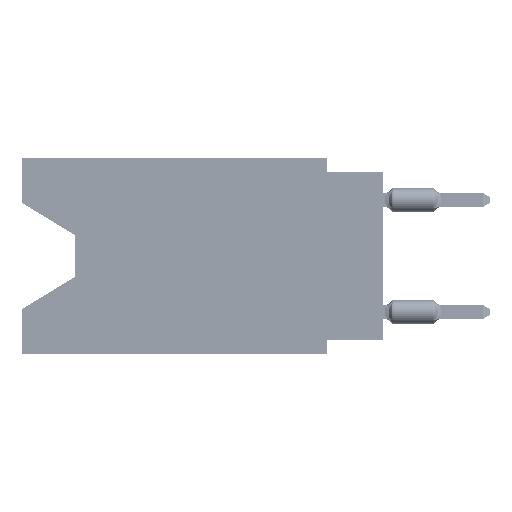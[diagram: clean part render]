
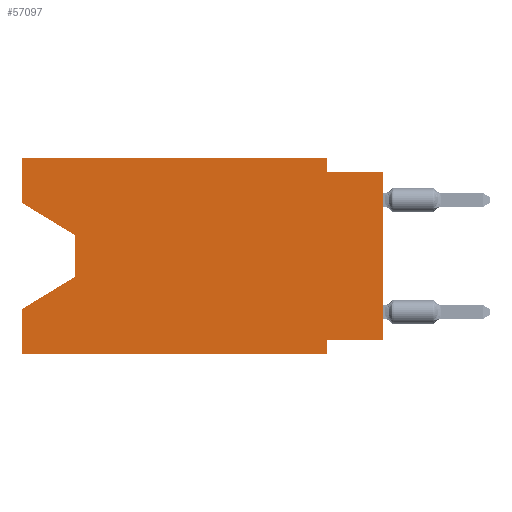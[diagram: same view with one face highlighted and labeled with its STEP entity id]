
A CAD part, left-side view. The second image highlights one B-rep face of the part: STEP entity #57097.
In plain terms, the highlighted planar face has unit normal (-1, 0, 0).
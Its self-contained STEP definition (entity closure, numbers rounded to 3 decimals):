
#537 = CARTESIAN_POINT ( 'NONE',  ( 0., 16.383, 0. ) ) ;
#1119 = VERTEX_POINT ( 'NONE', #93878 ) ;
#1334 = EDGE_CURVE ( 'NONE', #93852, #103266, #5822, .T. ) ;
#1930 = CARTESIAN_POINT ( 'NONE',  ( 0., 16.383, 0. ) ) ;
#2427 = LINE ( 'NONE', #102620, #50408 ) ;
#5214 = CARTESIAN_POINT ( 'NONE',  ( 0., 0., -0.635 ) ) ;
#5822 = LINE ( 'NONE', #48983, #24783 ) ;
#6375 = DIRECTION ( 'NONE',  ( 0., 0., -1. ) ) ;
#7652 = CARTESIAN_POINT ( 'NONE',  ( 0., 16.383, 0. ) ) ;
#9685 = DIRECTION ( 'NONE',  ( 0., 0., 1. ) ) ;
#10869 = CARTESIAN_POINT ( 'NONE',  ( 0., 16.383, -8.89 ) ) ;
#11173 = LINE ( 'NONE', #78660, #77022 ) ;
#13385 = DIRECTION ( 'NONE',  ( 0., 0.855, -0.519 ) ) ;
#14281 = EDGE_CURVE ( 'NONE', #69704, #1119, #11173, .T. ) ;
#15565 = CARTESIAN_POINT ( 'NONE',  ( 0., 13.97, -5.385 ) ) ;
#17592 = CARTESIAN_POINT ( 'NONE',  ( 0., 0., 0. ) ) ;
#18024 = CARTESIAN_POINT ( 'NONE',  ( 0., 2.54, -8.255 ) ) ;
#20036 = CARTESIAN_POINT ( 'NONE',  ( 0., 16.383, -8.89 ) ) ;
#22948 = EDGE_CURVE ( 'NONE', #95150, #103266, #60138, .T. ) ;
#24783 = VECTOR ( 'NONE', #6375, 1000. ) ;
#25630 = VECTOR ( 'NONE', #101150, 1000. ) ;
#25747 = ORIENTED_EDGE ( 'NONE', *, *, #84542, .F. ) ;
#26846 = FACE_OUTER_BOUND ( 'NONE', #79437, .T. ) ;
#29941 = DIRECTION ( 'NONE',  ( 0., 1., 0. ) ) ;
#30631 = CARTESIAN_POINT ( 'NONE',  ( 0., 16.383, 0. ) ) ;
#34101 = VERTEX_POINT ( 'NONE', #54511 ) ;
#35031 = DIRECTION ( 'NONE',  ( 0., 0., -1. ) ) ;
#36302 = VECTOR ( 'NONE', #53374, 1000. ) ;
#37730 = ORIENTED_EDGE ( 'NONE', *, *, #86153, .T. ) ;
#38272 = ORIENTED_EDGE ( 'NONE', *, *, #1334, .F. ) ;
#39080 = VERTEX_POINT ( 'NONE', #102708 ) ;
#39469 = ORIENTED_EDGE ( 'NONE', *, *, #47009, .F. ) ;
#40751 = VERTEX_POINT ( 'NONE', #79932 ) ;
#41187 = EDGE_CURVE ( 'NONE', #86800, #39080, #69320, .T. ) ;
#41399 = LINE ( 'NONE', #7652, #25630 ) ;
#43042 = ORIENTED_EDGE ( 'NONE', *, *, #75355, .F. ) ;
#43188 = EDGE_CURVE ( 'NONE', #34101, #86800, #80638, .T. ) ;
#44142 = CARTESIAN_POINT ( 'NONE',  ( 0., 2.54, 0. ) ) ;
#46734 = EDGE_CURVE ( 'NONE', #65352, #93852, #2427, .T. ) ;
#47009 = EDGE_CURVE ( 'NONE', #1119, #68268, #53933, .T. ) ;
#48882 = ORIENTED_EDGE ( 'NONE', *, *, #107267, .T. ) ;
#48983 = CARTESIAN_POINT ( 'NONE',  ( 0., 2.54, -8.89 ) ) ;
#50369 = DIRECTION ( 'NONE',  ( 0., 0., 1. ) ) ;
#50408 = VECTOR ( 'NONE', #29941, 1000. ) ;
#50520 = CARTESIAN_POINT ( 'NONE',  ( 0., 2.54, -8.89 ) ) ;
#50804 = DIRECTION ( 'NONE',  ( 0., 0., 1. ) ) ;
#51018 = CARTESIAN_POINT ( 'NONE',  ( 0., 13.97, -3.505 ) ) ;
#52054 = AXIS2_PLACEMENT_3D ( 'NONE', #1930, #67821, #84976 ) ;
#52733 = ORIENTED_EDGE ( 'NONE', *, *, #41187, .T. ) ;
#53374 = DIRECTION ( 'NONE',  ( 0., -1., 0. ) ) ;
#53933 = LINE ( 'NONE', #5214, #36302 ) ;
#54495 = ORIENTED_EDGE ( 'NONE', *, *, #43188, .T. ) ;
#54511 = CARTESIAN_POINT ( 'NONE',  ( 0., 16.383, -2.038 ) ) ;
#55204 = CARTESIAN_POINT ( 'NONE',  ( 0., 16.383, -2.038 ) ) ;
#57097 = ADVANCED_FACE ( 'NONE', ( #26846 ), #86041, .F. ) ;
#59106 = LINE ( 'NONE', #17592, #79151 ) ;
#60106 = ORIENTED_EDGE ( 'NONE', *, *, #79521, .F. ) ;
#60138 = LINE ( 'NONE', #10869, #65700 ) ;
#62964 = DIRECTION ( 'NONE',  ( 0., -0.855, -0.519 ) ) ;
#65352 = VERTEX_POINT ( 'NONE', #67817 ) ;
#65700 = VECTOR ( 'NONE', #68968, 1000. ) ;
#67817 = CARTESIAN_POINT ( 'NONE',  ( 0., 0., -8.255 ) ) ;
#67821 = DIRECTION ( 'NONE',  ( 1., 0., 0. ) ) ;
#68268 = VERTEX_POINT ( 'NONE', #68596 ) ;
#68596 = CARTESIAN_POINT ( 'NONE',  ( 0., 0., -0.635 ) ) ;
#68968 = DIRECTION ( 'NONE',  ( 0., -1., 0. ) ) ;
#69320 = LINE ( 'NONE', #103082, #72740 ) ;
#69704 = VERTEX_POINT ( 'NONE', #44142 ) ;
#70362 = DIRECTION ( 'NONE',  ( 0., 0., -1. ) ) ;
#72740 = VECTOR ( 'NONE', #35031, 1000. ) ;
#74940 = VECTOR ( 'NONE', #9685, 1000. ) ;
#75355 = EDGE_CURVE ( 'NONE', #76079, #69704, #41399, .T. ) ;
#76079 = VERTEX_POINT ( 'NONE', #30631 ) ;
#76090 = VECTOR ( 'NONE', #13385, 1000. ) ;
#77022 = VECTOR ( 'NONE', #70362, 1000. ) ;
#77391 = LINE ( 'NONE', #537, #96632 ) ;
#78660 = CARTESIAN_POINT ( 'NONE',  ( 0., 2.54, 0. ) ) ;
#79151 = VECTOR ( 'NONE', #50804, 1000. ) ;
#79437 = EDGE_LOOP ( 'NONE', ( #54495, #52733, #48882, #60106, #79614, #38272, #90159, #37730, #39469, #94304, #43042, #25747 ) ) ;
#79521 = EDGE_CURVE ( 'NONE', #95150, #40751, #93791, .T. ) ;
#79614 = ORIENTED_EDGE ( 'NONE', *, *, #22948, .T. ) ;
#79932 = CARTESIAN_POINT ( 'NONE',  ( 0., 16.383, -6.852 ) ) ;
#80638 = LINE ( 'NONE', #55204, #90679 ) ;
#84542 = EDGE_CURVE ( 'NONE', #34101, #76079, #77391, .T. ) ;
#84976 = DIRECTION ( 'NONE',  ( 0., 0., -1. ) ) ;
#85471 = CARTESIAN_POINT ( 'NONE',  ( 0., 16.383, 0. ) ) ;
#86041 = PLANE ( 'NONE',  #52054 ) ;
#86153 = EDGE_CURVE ( 'NONE', #65352, #68268, #59106, .T. ) ;
#86800 = VERTEX_POINT ( 'NONE', #51018 ) ;
#90159 = ORIENTED_EDGE ( 'NONE', *, *, #46734, .F. ) ;
#90679 = VECTOR ( 'NONE', #62964, 1000. ) ;
#91363 = LINE ( 'NONE', #15565, #76090 ) ;
#93791 = LINE ( 'NONE', #85471, #74940 ) ;
#93852 = VERTEX_POINT ( 'NONE', #18024 ) ;
#93878 = CARTESIAN_POINT ( 'NONE',  ( 0., 2.54, -0.635 ) ) ;
#94304 = ORIENTED_EDGE ( 'NONE', *, *, #14281, .F. ) ;
#95150 = VERTEX_POINT ( 'NONE', #20036 ) ;
#96632 = VECTOR ( 'NONE', #50369, 1000. ) ;
#101150 = DIRECTION ( 'NONE',  ( 0., -1., 0. ) ) ;
#102620 = CARTESIAN_POINT ( 'NONE',  ( 0., 0., -8.255 ) ) ;
#102708 = CARTESIAN_POINT ( 'NONE',  ( 0., 13.97, -5.385 ) ) ;
#103082 = CARTESIAN_POINT ( 'NONE',  ( 0., 13.97, -3.505 ) ) ;
#103266 = VERTEX_POINT ( 'NONE', #50520 ) ;
#107267 = EDGE_CURVE ( 'NONE', #39080, #40751, #91363, .T. ) ;
